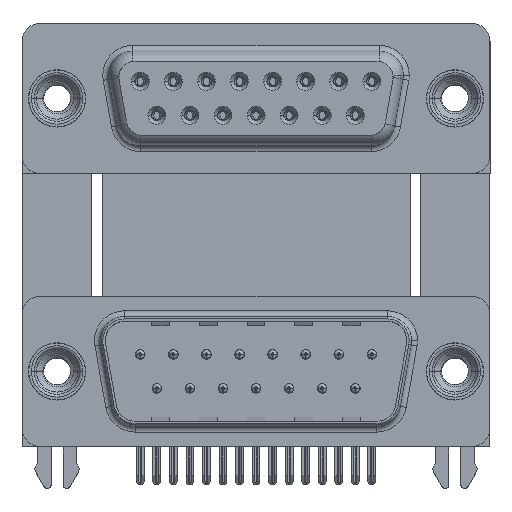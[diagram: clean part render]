
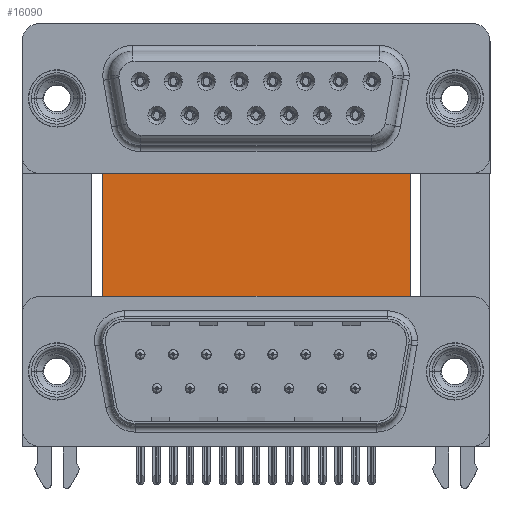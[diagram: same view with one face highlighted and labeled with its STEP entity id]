
A CAD part, top view. The second image highlights one B-rep face of the part: STEP entity #16090.
In plain terms, the highlighted planar face has unit normal (0, 0, 1).
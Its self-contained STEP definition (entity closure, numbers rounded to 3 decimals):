
#1116 = FACE_OUTER_BOUND ( 'NONE', #11574, .T. ) ;
#4254 = ORIENTED_EDGE ( 'NONE', *, *, #37941, .T. ) ;
#4675 = LINE ( 'NONE', #29895, #35012 ) ;
#5839 = CARTESIAN_POINT ( 'NONE',  ( 3.79, 16.585, -12. ) ) ;
#6900 = VERTEX_POINT ( 'NONE', #34774 ) ;
#7142 = VERTEX_POINT ( 'NONE', #26155 ) ;
#8214 = DIRECTION ( 'NONE',  ( 1., 0., 0. ) ) ;
#8820 = EDGE_CURVE ( 'NONE', #7142, #6900, #4675, .T. ) ;
#8896 = EDGE_CURVE ( 'NONE', #26058, #6900, #29655, .T. ) ;
#11574 = EDGE_LOOP ( 'NONE', ( #14487, #34930, #30315, #4254 ) ) ;
#11767 = CARTESIAN_POINT ( 'NONE',  ( 3.79, -3.735, -12. ) ) ;
#13814 = PLANE ( 'NONE',  #23672 ) ;
#14487 = ORIENTED_EDGE ( 'NONE', *, *, #8896, .T. ) ;
#16090 = ADVANCED_FACE ( 'NONE', ( #1116 ), #13814, .F. ) ;
#16109 = EDGE_CURVE ( 'NONE', #21175, #7142, #30791, .T. ) ;
#17109 = DIRECTION ( 'NONE',  ( -1., 0., 0. ) ) ;
#17352 = DIRECTION ( 'NONE',  ( 1., 0., 0. ) ) ;
#17711 = LINE ( 'NONE', #46476, #33809 ) ;
#19958 = CARTESIAN_POINT ( 'NONE',  ( 3.79, 16.585, -12. ) ) ;
#20663 = VECTOR ( 'NONE', #17352, 1000. ) ;
#21175 = VERTEX_POINT ( 'NONE', #5839 ) ;
#23672 = AXIS2_PLACEMENT_3D ( 'NONE', #27474, #31715, #17109 ) ;
#25002 = DIRECTION ( 'NONE',  ( 0., -1., 0. ) ) ;
#26058 = VERTEX_POINT ( 'NONE', #45235 ) ;
#26155 = CARTESIAN_POINT ( 'NONE',  ( 29.58, 16.585, -12. ) ) ;
#27474 = CARTESIAN_POINT ( 'NONE',  ( 3.79, 16.585, -12. ) ) ;
#27510 = VECTOR ( 'NONE', #8214, 1000. ) ;
#29655 = LINE ( 'NONE', #11767, #27510 ) ;
#29895 = CARTESIAN_POINT ( 'NONE',  ( 29.58, 16.585, -12. ) ) ;
#30315 = ORIENTED_EDGE ( 'NONE', *, *, #16109, .F. ) ;
#30791 = LINE ( 'NONE', #19958, #20663 ) ;
#31715 = DIRECTION ( 'NONE',  ( 0., 0., -1. ) ) ;
#32952 = DIRECTION ( 'NONE',  ( 0., -1., 0. ) ) ;
#33809 = VECTOR ( 'NONE', #25002, 1000. ) ;
#34774 = CARTESIAN_POINT ( 'NONE',  ( 29.58, -3.735, -12. ) ) ;
#34930 = ORIENTED_EDGE ( 'NONE', *, *, #8820, .F. ) ;
#35012 = VECTOR ( 'NONE', #32952, 1000. ) ;
#37941 = EDGE_CURVE ( 'NONE', #21175, #26058, #17711, .T. ) ;
#45235 = CARTESIAN_POINT ( 'NONE',  ( 3.79, -3.735, -12. ) ) ;
#46476 = CARTESIAN_POINT ( 'NONE',  ( 3.79, 16.585, -12. ) ) ;
